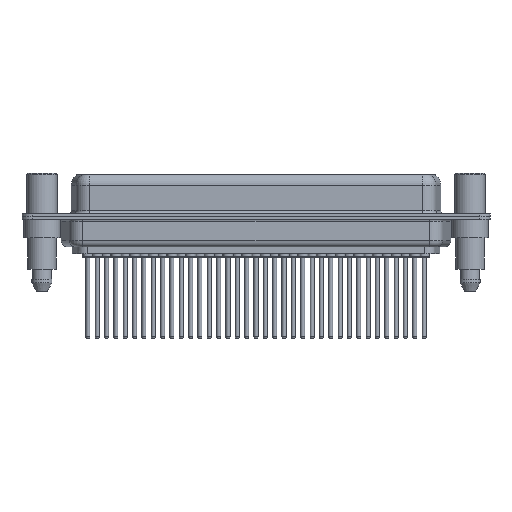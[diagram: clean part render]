
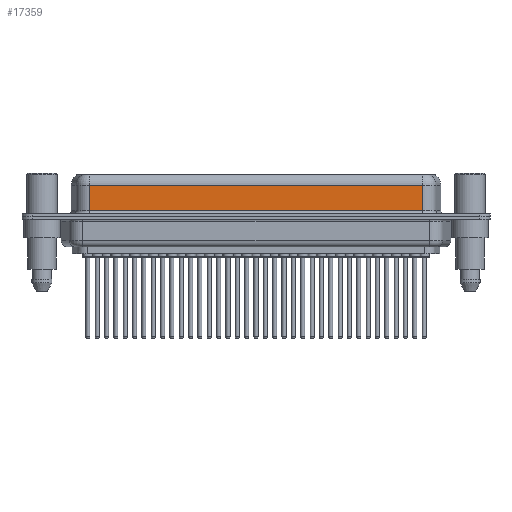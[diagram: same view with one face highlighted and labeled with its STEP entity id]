
A CAD part, front view. The second image highlights one B-rep face of the part: STEP entity #17359.
In plain terms, the highlighted planar face has unit normal (0, -1, 0).
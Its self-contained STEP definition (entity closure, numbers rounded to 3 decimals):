
#556 = PLANE ( 'NONE',  #20529 ) ;
#704 = DIRECTION ( 'NONE',  ( -1., 0., 0. ) ) ;
#2514 = VERTEX_POINT ( 'NONE', #26348 ) ;
#2662 = ORIENTED_EDGE ( 'NONE', *, *, #25327, .T. ) ;
#3017 = FACE_OUTER_BOUND ( 'NONE', #7782, .T. ) ;
#4461 = VECTOR ( 'NONE', #11041, 1000. ) ;
#4792 = ORIENTED_EDGE ( 'NONE', *, *, #8104, .T. ) ;
#5345 = CARTESIAN_POINT ( 'NONE',  ( 56.462, -3.95, 4.65 ) ) ;
#5824 = LINE ( 'NONE', #7992, #20075 ) ;
#6408 = DIRECTION ( 'NONE',  ( 0., 1., 0. ) ) ;
#6805 = VERTEX_POINT ( 'NONE', #5345 ) ;
#7288 = CARTESIAN_POINT ( 'NONE',  ( 7.038, -3.95, 6.4 ) ) ;
#7382 = LINE ( 'NONE', #9289, #4461 ) ;
#7782 = EDGE_LOOP ( 'NONE', ( #25830, #2662, #4792, #19905 ) ) ;
#7992 = CARTESIAN_POINT ( 'NONE',  ( 56.462, -3.95, 0.9 ) ) ;
#8104 = EDGE_CURVE ( 'NONE', #2514, #9744, #15870, .T. ) ;
#8862 = CARTESIAN_POINT ( 'NONE',  ( 7.038, -3.95, 0.9 ) ) ;
#9196 = EDGE_CURVE ( 'NONE', #9744, #26628, #5824, .T. ) ;
#9289 = CARTESIAN_POINT ( 'NONE',  ( 56.462, -3.95, 6.4 ) ) ;
#9744 = VERTEX_POINT ( 'NONE', #8862 ) ;
#11041 = DIRECTION ( 'NONE',  ( 0., 0., -1. ) ) ;
#11195 = VECTOR ( 'NONE', #20113, 1000. ) ;
#12067 = DIRECTION ( 'NONE',  ( 1., 0., 0. ) ) ;
#13512 = DIRECTION ( 'NONE',  ( -1., 0., 0. ) ) ;
#14840 = CARTESIAN_POINT ( 'NONE',  ( 56.462, -3.95, 6.4 ) ) ;
#15560 = LINE ( 'NONE', #25700, #22352 ) ;
#15870 = LINE ( 'NONE', #7288, #11195 ) ;
#17359 = ADVANCED_FACE ( 'NONE', ( #3017 ), #556, .F. ) ;
#18982 = CARTESIAN_POINT ( 'NONE',  ( 56.462, -3.95, 0.9 ) ) ;
#19905 = ORIENTED_EDGE ( 'NONE', *, *, #9196, .T. ) ;
#20075 = VECTOR ( 'NONE', #12067, 1000. ) ;
#20113 = DIRECTION ( 'NONE',  ( 0., 0., -1. ) ) ;
#20529 = AXIS2_PLACEMENT_3D ( 'NONE', #14840, #6408, #704 ) ;
#22352 = VECTOR ( 'NONE', #13512, 1000. ) ;
#25327 = EDGE_CURVE ( 'NONE', #6805, #2514, #15560, .T. ) ;
#25700 = CARTESIAN_POINT ( 'NONE',  ( 56.462, -3.95, 4.65 ) ) ;
#25830 = ORIENTED_EDGE ( 'NONE', *, *, #26777, .F. ) ;
#26348 = CARTESIAN_POINT ( 'NONE',  ( 7.038, -3.95, 4.65 ) ) ;
#26628 = VERTEX_POINT ( 'NONE', #18982 ) ;
#26777 = EDGE_CURVE ( 'NONE', #6805, #26628, #7382, .T. ) ;
